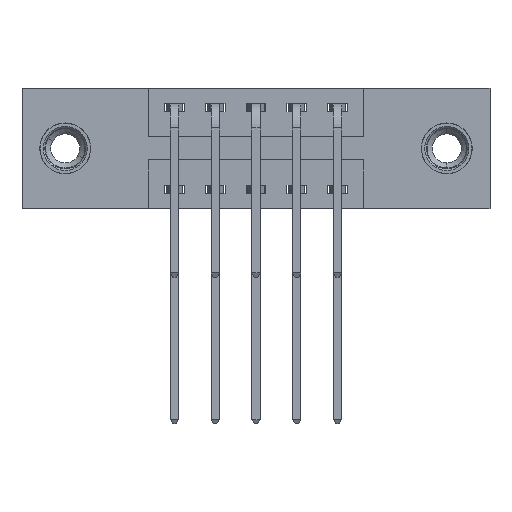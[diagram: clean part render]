
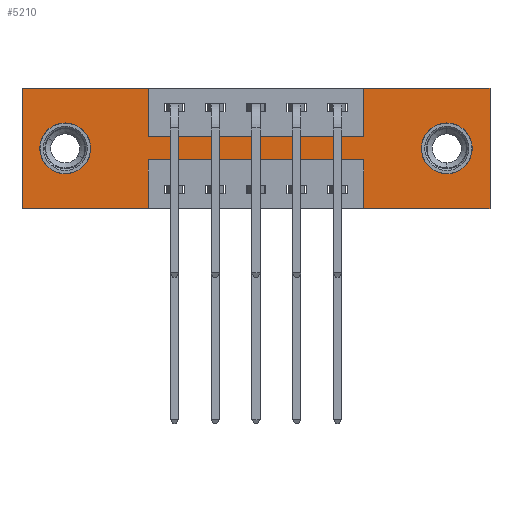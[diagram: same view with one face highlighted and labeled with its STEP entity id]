
A CAD part, front view. The second image highlights one B-rep face of the part: STEP entity #5210.
In plain terms, the highlighted planar face has unit normal (0, -1, 0).
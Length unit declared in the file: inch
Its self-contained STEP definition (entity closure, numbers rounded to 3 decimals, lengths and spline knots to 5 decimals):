
#215 = ORIENTED_EDGE ( 'NONE', *, *, #7693, .F. ) ;
#291 = ORIENTED_EDGE ( 'NONE', *, *, #7611, .F. ) ;
#355 = VERTEX_POINT ( 'NONE', #11032 ) ;
#439 = CARTESIAN_POINT ( 'NONE',  ( 1.435, 0., 0. ) ) ;
#511 = ORIENTED_EDGE ( 'NONE', *, *, #7708, .F. ) ;
#512 = EDGE_LOOP ( 'NONE', ( #3467, #11185, #291, #1324, #9428, #2247, #3644, #215, #511, #1579, #2230, #2303 ) ) ;
#672 = VERTEX_POINT ( 'NONE', #3016 ) ;
#769 = VERTEX_POINT ( 'NONE', #439 ) ;
#908 = DIRECTION ( 'NONE',  ( 0., 0., -1. ) ) ;
#1016 = EDGE_LOOP ( 'NONE', ( #7057, #7320 ) ) ;
#1084 = CARTESIAN_POINT ( 'NONE',  ( 0.3875, 0., -0.37 ) ) ;
#1137 = DIRECTION ( 'NONE',  ( 0., 0., -1. ) ) ;
#1160 = DIRECTION ( 'NONE',  ( 1., 0., 0. ) ) ;
#1187 = CARTESIAN_POINT ( 'NONE',  ( 0., 0., 0. ) ) ;
#1261 = VERTEX_POINT ( 'NONE', #8952 ) ;
#1274 = VERTEX_POINT ( 'NONE', #8893 ) ;
#1324 = ORIENTED_EDGE ( 'NONE', *, *, #6797, .F. ) ;
#1483 = CARTESIAN_POINT ( 'NONE',  ( 1.0475, 0., -0.22 ) ) ;
#1507 = CARTESIAN_POINT ( 'NONE',  ( 1.435, 0., 0. ) ) ;
#1579 = ORIENTED_EDGE ( 'NONE', *, *, #2318, .F. ) ;
#1609 = DIRECTION ( 'NONE',  ( 0., 1., 0. ) ) ;
#1625 = LINE ( 'NONE', #5677, #10020 ) ;
#1626 = DIRECTION ( 'NONE',  ( 0., 0., 1. ) ) ;
#1638 = VECTOR ( 'NONE', #3000, 39.37008 ) ;
#1646 = DIRECTION ( 'NONE',  ( 1., 0., 0. ) ) ;
#1667 = CARTESIAN_POINT ( 'NONE',  ( 0., 0., 0. ) ) ;
#1689 = CARTESIAN_POINT ( 'NONE',  ( 0.1325, 0., -0.185 ) ) ;
#1980 = DIRECTION ( 'NONE',  ( 0., 0., -1. ) ) ;
#1995 = DIRECTION ( 'NONE',  ( 0., -1., 0. ) ) ;
#2009 = CARTESIAN_POINT ( 'NONE',  ( 0., 0., -0.37 ) ) ;
#2047 = VERTEX_POINT ( 'NONE', #4397 ) ;
#2049 = PLANE ( 'NONE',  #8891 ) ;
#2079 = CARTESIAN_POINT ( 'NONE',  ( 1.435, 0., -0.37 ) ) ;
#2151 = CIRCLE ( 'NONE', #6168, 0.078 ) ;
#2186 = DIRECTION ( 'NONE',  ( 0., 0., -1. ) ) ;
#2230 = ORIENTED_EDGE ( 'NONE', *, *, #6443, .F. ) ;
#2247 = ORIENTED_EDGE ( 'NONE', *, *, #2374, .F. ) ;
#2287 = CARTESIAN_POINT ( 'NONE',  ( 1.3025, 0., -0.185 ) ) ;
#2303 = ORIENTED_EDGE ( 'NONE', *, *, #6974, .F. ) ;
#2311 = FACE_OUTER_BOUND ( 'NONE', #512, .T. ) ;
#2318 = EDGE_CURVE ( 'NONE', #672, #2047, #6238, .T. ) ;
#2361 = VECTOR ( 'NONE', #2549, 39.37008 ) ;
#2374 = EDGE_CURVE ( 'NONE', #355, #769, #5948, .T. ) ;
#2380 = DIRECTION ( 'NONE',  ( 0., 1., 0. ) ) ;
#2396 = CARTESIAN_POINT ( 'NONE',  ( 0., 0., 0. ) ) ;
#2479 = FACE_BOUND ( 'NONE', #1016, .T. ) ;
#2549 = DIRECTION ( 'NONE',  ( 0., 0., 1. ) ) ;
#2881 = FACE_BOUND ( 'NONE', #11232, .T. ) ;
#2943 = EDGE_CURVE ( 'NONE', #10848, #8060, #4538, .T. ) ;
#2964 = LINE ( 'NONE', #2396, #2361 ) ;
#3000 = DIRECTION ( 'NONE',  ( -1., 0., 0. ) ) ;
#3016 = CARTESIAN_POINT ( 'NONE',  ( 0., 0., 0. ) ) ;
#3070 = CARTESIAN_POINT ( 'NONE',  ( 1.0475, 0., -0.37 ) ) ;
#3118 = DIRECTION ( 'NONE',  ( -1., 0., 0. ) ) ;
#3253 = DIRECTION ( 'NONE',  ( 0., 0., -1. ) ) ;
#3467 = ORIENTED_EDGE ( 'NONE', *, *, #7563, .F. ) ;
#3644 = ORIENTED_EDGE ( 'NONE', *, *, #7677, .F. ) ;
#3649 = EDGE_CURVE ( 'NONE', #11240, #1261, #2151, .T. ) ;
#3903 = ORIENTED_EDGE ( 'NONE', *, *, #2943, .T. ) ;
#4014 = VECTOR ( 'NONE', #3253, 39.37008 ) ;
#4036 = VECTOR ( 'NONE', #908, 39.37008 ) ;
#4154 = CARTESIAN_POINT ( 'NONE',  ( 1.0475, 0., -0.15 ) ) ;
#4175 = CARTESIAN_POINT ( 'NONE',  ( 0.3875, 0., -0.15 ) ) ;
#4301 = DIRECTION ( 'NONE',  ( 0., 0., 1. ) ) ;
#4303 = DIRECTION ( 'NONE',  ( 0., 1., 0. ) ) ;
#4317 = CARTESIAN_POINT ( 'NONE',  ( 0.1325, 0., -0.185 ) ) ;
#4397 = CARTESIAN_POINT ( 'NONE',  ( 0.3875, 0., 0. ) ) ;
#4538 = CIRCLE ( 'NONE', #9411, 0.078 ) ;
#4838 = VERTEX_POINT ( 'NONE', #5490 ) ;
#4990 = EDGE_CURVE ( 'NONE', #8060, #10848, #9059, .T. ) ;
#5019 = VERTEX_POINT ( 'NONE', #4154 ) ;
#5130 = LINE ( 'NONE', #9973, #9263 ) ;
#5210 = ADVANCED_FACE ( 'NONE', ( #2479, #2881, #2311 ), #2049, .T. ) ;
#5371 = VECTOR ( 'NONE', #7255, 39.37008 ) ;
#5446 = CARTESIAN_POINT ( 'NONE',  ( 1.3025, 0., -0.185 ) ) ;
#5490 = CARTESIAN_POINT ( 'NONE',  ( 0.3875, 0., -0.22 ) ) ;
#5677 = CARTESIAN_POINT ( 'NONE',  ( 0.3875, 0., -0.37 ) ) ;
#5914 = VECTOR ( 'NONE', #1160, 39.37008 ) ;
#5948 = LINE ( 'NONE', #1187, #5914 ) ;
#6168 = AXIS2_PLACEMENT_3D ( 'NONE', #2287, #2380, #2186 ) ;
#6178 = VECTOR ( 'NONE', #1646, 39.37008 ) ;
#6199 = DIRECTION ( 'NONE',  ( 0., 0., -1. ) ) ;
#6238 = LINE ( 'NONE', #1667, #6178 ) ;
#6299 = CARTESIAN_POINT ( 'NONE',  ( 0.1325, 0., -0.263 ) ) ;
#6328 = LINE ( 'NONE', #9824, #1638 ) ;
#6443 = EDGE_CURVE ( 'NONE', #9457, #672, #2964, .T. ) ;
#6455 = CARTESIAN_POINT ( 'NONE',  ( 0.3875, 0., -0.22 ) ) ;
#6555 = EDGE_CURVE ( 'NONE', #769, #6809, #10622, .T. ) ;
#6580 = CARTESIAN_POINT ( 'NONE',  ( 1.0475, 0., 0. ) ) ;
#6658 = CARTESIAN_POINT ( 'NONE',  ( 1.0475, 0., -0.37 ) ) ;
#6797 = EDGE_CURVE ( 'NONE', #6809, #10712, #6328, .T. ) ;
#6809 = VERTEX_POINT ( 'NONE', #2079 ) ;
#6934 = LINE ( 'NONE', #6580, #8978 ) ;
#6974 = EDGE_CURVE ( 'NONE', #8188, #9457, #5130, .T. ) ;
#7057 = ORIENTED_EDGE ( 'NONE', *, *, #7359, .T. ) ;
#7255 = DIRECTION ( 'NONE',  ( -1., 0., 0. ) ) ;
#7285 = CARTESIAN_POINT ( 'NONE',  ( 1.3025, 0., -0.263 ) ) ;
#7320 = ORIENTED_EDGE ( 'NONE', *, *, #3649, .T. ) ;
#7359 = EDGE_CURVE ( 'NONE', #1261, #11240, #8573, .T. ) ;
#7413 = DIRECTION ( 'NONE',  ( 1., 0., 0. ) ) ;
#7465 = LINE ( 'NONE', #6455, #5371 ) ;
#7563 = EDGE_CURVE ( 'NONE', #4838, #8188, #1625, .T. ) ;
#7579 = EDGE_CURVE ( 'NONE', #9234, #4838, #7465, .T. ) ;
#7611 = EDGE_CURVE ( 'NONE', #10712, #9234, #7733, .T. ) ;
#7677 = EDGE_CURVE ( 'NONE', #5019, #355, #6934, .T. ) ;
#7693 = EDGE_CURVE ( 'NONE', #1274, #5019, #8702, .T. ) ;
#7708 = EDGE_CURVE ( 'NONE', #2047, #1274, #10603, .T. ) ;
#7733 = LINE ( 'NONE', #3070, #9755 ) ;
#7834 = CARTESIAN_POINT ( 'NONE',  ( 0., 0., -0.37 ) ) ;
#8060 = VERTEX_POINT ( 'NONE', #6299 ) ;
#8171 = DIRECTION ( 'NONE',  ( 0., 0., 1. ) ) ;
#8188 = VERTEX_POINT ( 'NONE', #1084 ) ;
#8234 = DIRECTION ( 'NONE',  ( 0., 0., 1. ) ) ;
#8313 = CARTESIAN_POINT ( 'NONE',  ( 0.3875, 0., 0. ) ) ;
#8413 = VECTOR ( 'NONE', #7413, 39.37008 ) ;
#8523 = CARTESIAN_POINT ( 'NONE',  ( 0.1325, 0., -0.107 ) ) ;
#8573 = CIRCLE ( 'NONE', #10561, 0.078 ) ;
#8702 = LINE ( 'NONE', #4175, #8413 ) ;
#8796 = AXIS2_PLACEMENT_3D ( 'NONE', #4317, #4303, #4301 ) ;
#8891 = AXIS2_PLACEMENT_3D ( 'NONE', #2009, #1995, #1980 ) ;
#8893 = CARTESIAN_POINT ( 'NONE',  ( 0.3875, 0., -0.15 ) ) ;
#8952 = CARTESIAN_POINT ( 'NONE',  ( 1.3025, 0., -0.107 ) ) ;
#8978 = VECTOR ( 'NONE', #8234, 39.37008 ) ;
#9059 = CIRCLE ( 'NONE', #8796, 0.078 ) ;
#9234 = VERTEX_POINT ( 'NONE', #1483 ) ;
#9263 = VECTOR ( 'NONE', #3118, 39.37008 ) ;
#9411 = AXIS2_PLACEMENT_3D ( 'NONE', #1689, #1609, #1626 ) ;
#9428 = ORIENTED_EDGE ( 'NONE', *, *, #6555, .F. ) ;
#9457 = VERTEX_POINT ( 'NONE', #7834 ) ;
#9755 = VECTOR ( 'NONE', #8171, 39.37008 ) ;
#9824 = CARTESIAN_POINT ( 'NONE',  ( 0., 0., -0.37 ) ) ;
#9925 = ORIENTED_EDGE ( 'NONE', *, *, #4990, .T. ) ;
#9973 = CARTESIAN_POINT ( 'NONE',  ( 0., 0., -0.37 ) ) ;
#10020 = VECTOR ( 'NONE', #1137, 39.37008 ) ;
#10561 = AXIS2_PLACEMENT_3D ( 'NONE', #5446, #11128, #6199 ) ;
#10603 = LINE ( 'NONE', #8313, #4014 ) ;
#10622 = LINE ( 'NONE', #1507, #4036 ) ;
#10712 = VERTEX_POINT ( 'NONE', #6658 ) ;
#10848 = VERTEX_POINT ( 'NONE', #8523 ) ;
#11032 = CARTESIAN_POINT ( 'NONE',  ( 1.0475, 0., 0. ) ) ;
#11128 = DIRECTION ( 'NONE',  ( 0., 1., 0. ) ) ;
#11185 = ORIENTED_EDGE ( 'NONE', *, *, #7579, .F. ) ;
#11232 = EDGE_LOOP ( 'NONE', ( #3903, #9925 ) ) ;
#11240 = VERTEX_POINT ( 'NONE', #7285 ) ;
